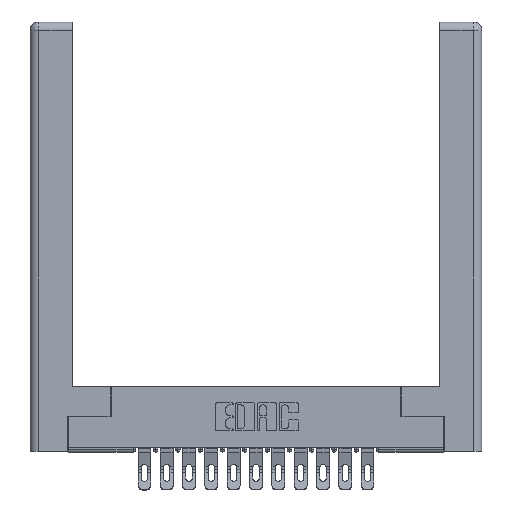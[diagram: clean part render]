
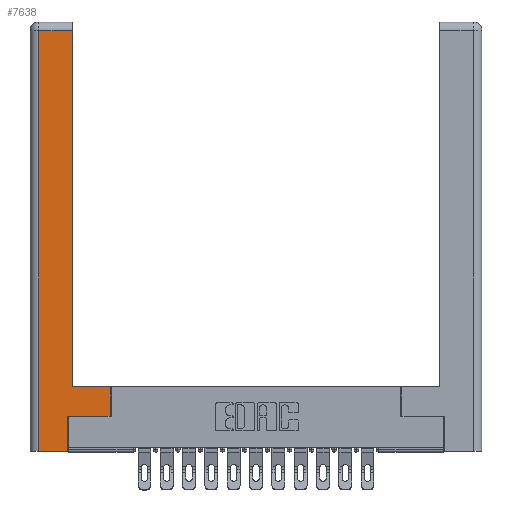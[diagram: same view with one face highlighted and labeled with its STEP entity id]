
A CAD part, top view. The second image highlights one B-rep face of the part: STEP entity #7638.
In plain terms, the highlighted planar face has unit normal (0, 0, 1).
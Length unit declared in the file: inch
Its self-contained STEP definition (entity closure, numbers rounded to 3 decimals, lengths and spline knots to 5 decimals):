
#220 = DIRECTION ( 'NONE',  ( 0., 1., 0. ) ) ;
#446 = CARTESIAN_POINT ( 'NONE',  ( 0.295, 0.45, 0. ) ) ;
#573 = VERTEX_POINT ( 'NONE', #3063 ) ;
#782 = LINE ( 'NONE', #6551, #10665 ) ;
#1815 = LINE ( 'NONE', #6628, #13259 ) ;
#2188 = VERTEX_POINT ( 'NONE', #3212 ) ;
#2464 = VERTEX_POINT ( 'NONE', #11841 ) ;
#2468 = LINE ( 'NONE', #3293, #4560 ) ;
#3063 = CARTESIAN_POINT ( 'NONE',  ( 0.565, 0.45, 0. ) ) ;
#3212 = CARTESIAN_POINT ( 'NONE',  ( 0.565, 0.245, 0. ) ) ;
#3293 = CARTESIAN_POINT ( 'NONE',  ( 0.265, 0., 0. ) ) ;
#3545 = VECTOR ( 'NONE', #11323, 39.37008 ) ;
#3856 = ORIENTED_EDGE ( 'NONE', *, *, #5728, .T. ) ;
#4217 = LINE ( 'NONE', #9517, #15389 ) ;
#4560 = VECTOR ( 'NONE', #7746, 39.37008 ) ;
#5126 = EDGE_LOOP ( 'NONE', ( #12244, #16356, #6621, #7620, #18843, #14990, #10626, #3856 ) ) ;
#5728 = EDGE_CURVE ( 'NONE', #573, #2464, #15789, .T. ) ;
#6089 = CARTESIAN_POINT ( 'NONE',  ( 0.295, 3., 0. ) ) ;
#6267 = PLANE ( 'NONE',  #13871 ) ;
#6538 = CARTESIAN_POINT ( 'NONE',  ( 0.265, 0.245, 0. ) ) ;
#6551 = CARTESIAN_POINT ( 'NONE',  ( 0.0615, 0., 0. ) ) ;
#6621 = ORIENTED_EDGE ( 'NONE', *, *, #13001, .T. ) ;
#6628 = CARTESIAN_POINT ( 'NONE',  ( 0.0615, 2.94, 0. ) ) ;
#6828 = LINE ( 'NONE', #6089, #7539 ) ;
#7307 = CARTESIAN_POINT ( 'NONE',  ( 0.265, 0.245, 0. ) ) ;
#7346 = EDGE_CURVE ( 'NONE', #9901, #16267, #15534, .T. ) ;
#7539 = VECTOR ( 'NONE', #220, 39.37008 ) ;
#7620 = ORIENTED_EDGE ( 'NONE', *, *, #10291, .T. ) ;
#7638 = ADVANCED_FACE ( 'NONE', ( #10577 ), #6267, .F. ) ;
#7682 = LINE ( 'NONE', #16892, #3545 ) ;
#7746 = DIRECTION ( 'NONE',  ( 1., 0., 0. ) ) ;
#9517 = CARTESIAN_POINT ( 'NONE',  ( 0.565, 0.45, 0. ) ) ;
#9520 = DIRECTION ( 'NONE',  ( 0., -1., 0. ) ) ;
#9901 = VERTEX_POINT ( 'NONE', #16941 ) ;
#10291 = EDGE_CURVE ( 'NONE', #16964, #9901, #2468, .T. ) ;
#10577 = FACE_OUTER_BOUND ( 'NONE', #5126, .T. ) ;
#10626 = ORIENTED_EDGE ( 'NONE', *, *, #12360, .T. ) ;
#10665 = VECTOR ( 'NONE', #9520, 39.37008 ) ;
#10733 = EDGE_CURVE ( 'NONE', #2464, #12164, #6828, .T. ) ;
#11046 = CARTESIAN_POINT ( 'NONE',  ( 0.295, 2.94, 0. ) ) ;
#11323 = DIRECTION ( 'NONE',  ( 1., 0., 0. ) ) ;
#11841 = CARTESIAN_POINT ( 'NONE',  ( 0.295, 0.45, 0. ) ) ;
#12123 = DIRECTION ( 'NONE',  ( 0., 0., -1. ) ) ;
#12141 = VECTOR ( 'NONE', #13729, 39.37008 ) ;
#12159 = CARTESIAN_POINT ( 'NONE',  ( 0.0615, 0., 0. ) ) ;
#12164 = VERTEX_POINT ( 'NONE', #11046 ) ;
#12244 = ORIENTED_EDGE ( 'NONE', *, *, #10733, .T. ) ;
#12290 = DIRECTION ( 'NONE',  ( -1., 0., 0. ) ) ;
#12360 = EDGE_CURVE ( 'NONE', #2188, #573, #4217, .T. ) ;
#12410 = DIRECTION ( 'NONE',  ( 0., 1., 0. ) ) ;
#13001 = EDGE_CURVE ( 'NONE', #14008, #16964, #782, .T. ) ;
#13026 = EDGE_CURVE ( 'NONE', #16267, #2188, #7682, .T. ) ;
#13259 = VECTOR ( 'NONE', #18283, 39.37008 ) ;
#13729 = DIRECTION ( 'NONE',  ( 0., 1., 0. ) ) ;
#13871 = AXIS2_PLACEMENT_3D ( 'NONE', #17910, #12123, #16491 ) ;
#14008 = VERTEX_POINT ( 'NONE', #14128 ) ;
#14128 = CARTESIAN_POINT ( 'NONE',  ( 0.0615, 2.94, 0. ) ) ;
#14990 = ORIENTED_EDGE ( 'NONE', *, *, #13026, .T. ) ;
#15303 = EDGE_CURVE ( 'NONE', #12164, #14008, #1815, .T. ) ;
#15389 = VECTOR ( 'NONE', #12410, 39.37008 ) ;
#15534 = LINE ( 'NONE', #6538, #12141 ) ;
#15789 = LINE ( 'NONE', #446, #18336 ) ;
#16267 = VERTEX_POINT ( 'NONE', #7307 ) ;
#16356 = ORIENTED_EDGE ( 'NONE', *, *, #15303, .T. ) ;
#16491 = DIRECTION ( 'NONE',  ( -1., 0., 0. ) ) ;
#16892 = CARTESIAN_POINT ( 'NONE',  ( 0.565, 0.245, 0. ) ) ;
#16941 = CARTESIAN_POINT ( 'NONE',  ( 0.265, 0., 0. ) ) ;
#16964 = VERTEX_POINT ( 'NONE', #12159 ) ;
#17910 = CARTESIAN_POINT ( 'NONE',  ( 0., 0., 0. ) ) ;
#18283 = DIRECTION ( 'NONE',  ( -1., 0., 0. ) ) ;
#18336 = VECTOR ( 'NONE', #12290, 39.37008 ) ;
#18843 = ORIENTED_EDGE ( 'NONE', *, *, #7346, .T. ) ;
